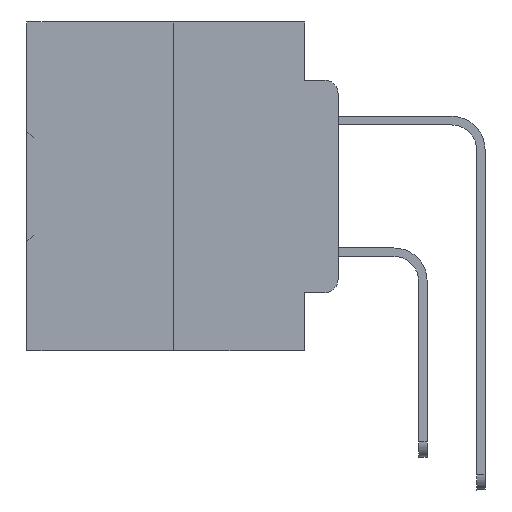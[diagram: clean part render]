
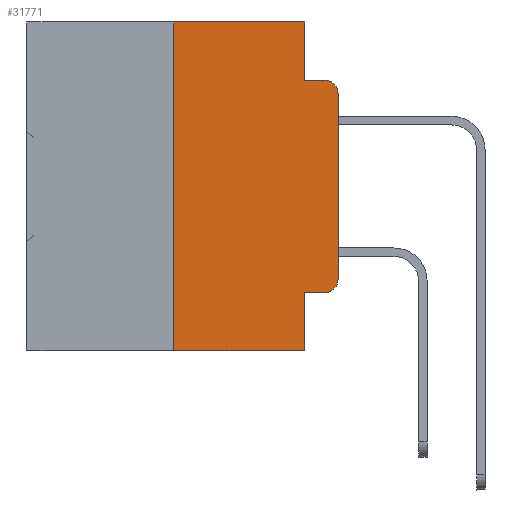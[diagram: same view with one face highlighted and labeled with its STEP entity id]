
A CAD part, left-side view. The second image highlights one B-rep face of the part: STEP entity #31771.
In plain terms, the highlighted planar face has unit normal (-1, 0, 0).
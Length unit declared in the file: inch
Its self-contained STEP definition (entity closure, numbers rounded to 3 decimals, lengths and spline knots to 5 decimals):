
#465 = LINE ( 'NONE', #18030, #31198 ) ;
#1318 = LINE ( 'NONE', #3230, #31983 ) ;
#2475 = DIRECTION ( 'NONE',  ( 0., 0., -1. ) ) ;
#2987 = EDGE_CURVE ( 'NONE', #26139, #19857, #32625, .T. ) ;
#3230 = CARTESIAN_POINT ( 'NONE',  ( 0., 0.25, 0. ) ) ;
#3264 = FACE_OUTER_BOUND ( 'NONE', #35237, .T. ) ;
#4497 = VERTEX_POINT ( 'NONE', #24549 ) ;
#4866 = ORIENTED_EDGE ( 'NONE', *, *, #21084, .F. ) ;
#6070 = DIRECTION ( 'NONE',  ( 0., 0., 1. ) ) ;
#6097 = CARTESIAN_POINT ( 'NONE',  ( 0., 0.051, -0.4115 ) ) ;
#6256 = DIRECTION ( 'NONE',  ( 0., -1., 0. ) ) ;
#6390 = CARTESIAN_POINT ( 'NONE',  ( 0., 0.473, -0.5 ) ) ;
#7211 = ORIENTED_EDGE ( 'NONE', *, *, #20123, .F. ) ;
#7515 = AXIS2_PLACEMENT_3D ( 'NONE', #36043, #9450, #29818 ) ;
#7609 = VECTOR ( 'NONE', #23160, 39.37008 ) ;
#8146 = ORIENTED_EDGE ( 'NONE', *, *, #8311, .F. ) ;
#8180 = LINE ( 'NONE', #6390, #29022 ) ;
#8311 = EDGE_CURVE ( 'NONE', #30500, #19254, #32648, .T. ) ;
#9120 = DIRECTION ( 'NONE',  ( 0., -1., 0. ) ) ;
#9134 = VECTOR ( 'NONE', #10815, 39.37008 ) ;
#9450 = DIRECTION ( 'NONE',  ( -1., 0., 0. ) ) ;
#10042 = ORIENTED_EDGE ( 'NONE', *, *, #34642, .F. ) ;
#10246 = CARTESIAN_POINT ( 'NONE',  ( 0., 0.051, -0.4115 ) ) ;
#10800 = VERTEX_POINT ( 'NONE', #15929 ) ;
#10815 = DIRECTION ( 'NONE',  ( 0., 0., -1. ) ) ;
#12585 = DIRECTION ( 'NONE',  ( 0., -1., 0. ) ) ;
#12762 = CIRCLE ( 'NONE', #13317, 0.02 ) ;
#12876 = ORIENTED_EDGE ( 'NONE', *, *, #13120, .T. ) ;
#13120 = EDGE_CURVE ( 'NONE', #19625, #26139, #36377, .T. ) ;
#13194 = DIRECTION ( 'NONE',  ( -1., 0., 0. ) ) ;
#13317 = AXIS2_PLACEMENT_3D ( 'NONE', #30758, #13194, #33690 ) ;
#13896 = VERTEX_POINT ( 'NONE', #32907 ) ;
#14576 = CARTESIAN_POINT ( 'NONE',  ( 0., 0.02, -0.4115 ) ) ;
#14990 = VECTOR ( 'NONE', #12585, 39.37008 ) ;
#15929 = CARTESIAN_POINT ( 'NONE',  ( 0., 0.051, -0.5 ) ) ;
#18030 = CARTESIAN_POINT ( 'NONE',  ( 0., 0., 0. ) ) ;
#18532 = CARTESIAN_POINT ( 'NONE',  ( 0., 0.02, -0.0885 ) ) ;
#19254 = VERTEX_POINT ( 'NONE', #26486 ) ;
#19493 = VECTOR ( 'NONE', #24830, 39.37008 ) ;
#19625 = VERTEX_POINT ( 'NONE', #10246 ) ;
#19795 = VERTEX_POINT ( 'NONE', #28828 ) ;
#19857 = VERTEX_POINT ( 'NONE', #32105 ) ;
#20123 = EDGE_CURVE ( 'NONE', #19254, #25121, #38294, .T. ) ;
#20477 = DIRECTION ( 'NONE',  ( 1., 0., 0. ) ) ;
#20642 = EDGE_CURVE ( 'NONE', #19857, #13896, #465, .T. ) ;
#21084 = EDGE_CURVE ( 'NONE', #19625, #10800, #31165, .T. ) ;
#23070 = EDGE_CURVE ( 'NONE', #19795, #4497, #1318, .T. ) ;
#23160 = DIRECTION ( 'NONE',  ( 0., 0., -1. ) ) ;
#24549 = CARTESIAN_POINT ( 'NONE',  ( 0., 0.25, 0. ) ) ;
#24830 = DIRECTION ( 'NONE',  ( 0., -1., 0. ) ) ;
#25121 = VERTEX_POINT ( 'NONE', #18532 ) ;
#25343 = AXIS2_PLACEMENT_3D ( 'NONE', #37882, #20477, #2475 ) ;
#25831 = CARTESIAN_POINT ( 'NONE',  ( 0., 0.051, 0. ) ) ;
#25849 = ORIENTED_EDGE ( 'NONE', *, *, #23070, .F. ) ;
#26139 = VERTEX_POINT ( 'NONE', #14576 ) ;
#26312 = EDGE_CURVE ( 'NONE', #19795, #10800, #8180, .T. ) ;
#26486 = CARTESIAN_POINT ( 'NONE',  ( 0., 0.051, -0.0885 ) ) ;
#27195 = ORIENTED_EDGE ( 'NONE', *, *, #20642, .T. ) ;
#27282 = LINE ( 'NONE', #30603, #19493 ) ;
#27302 = CARTESIAN_POINT ( 'NONE',  ( 0., 0.051, -0.0885 ) ) ;
#28070 = ORIENTED_EDGE ( 'NONE', *, *, #37670, .T. ) ;
#28828 = CARTESIAN_POINT ( 'NONE',  ( 0., 0.25, -0.5 ) ) ;
#29022 = VECTOR ( 'NONE', #6256, 39.37008 ) ;
#29818 = DIRECTION ( 'NONE',  ( 0., 0., -1. ) ) ;
#30500 = VERTEX_POINT ( 'NONE', #25831 ) ;
#30603 = CARTESIAN_POINT ( 'NONE',  ( 0., 0.473, 0. ) ) ;
#30758 = CARTESIAN_POINT ( 'NONE',  ( 0., 0.02, -0.1085 ) ) ;
#31165 = LINE ( 'NONE', #37603, #7609 ) ;
#31198 = VECTOR ( 'NONE', #6070, 39.37008 ) ;
#31391 = CARTESIAN_POINT ( 'NONE',  ( 0., 0.051, 0. ) ) ;
#31771 = ADVANCED_FACE ( 'NONE', ( #3264 ), #32039, .F. ) ;
#31983 = VECTOR ( 'NONE', #32881, 39.37008 ) ;
#32039 = PLANE ( 'NONE',  #25343 ) ;
#32105 = CARTESIAN_POINT ( 'NONE',  ( 0., 0., -0.3915 ) ) ;
#32625 = CIRCLE ( 'NONE', #7515, 0.02 ) ;
#32648 = LINE ( 'NONE', #31391, #9134 ) ;
#32881 = DIRECTION ( 'NONE',  ( 0., 0., 1. ) ) ;
#32907 = CARTESIAN_POINT ( 'NONE',  ( 0., 0., -0.1085 ) ) ;
#33505 = ORIENTED_EDGE ( 'NONE', *, *, #26312, .T. ) ;
#33690 = DIRECTION ( 'NONE',  ( 0., 0., -1. ) ) ;
#34642 = EDGE_CURVE ( 'NONE', #4497, #30500, #27282, .T. ) ;
#35237 = EDGE_LOOP ( 'NONE', ( #27195, #28070, #7211, #8146, #10042, #25849, #33505, #4866, #12876, #36250 ) ) ;
#35486 = VECTOR ( 'NONE', #9120, 39.37008 ) ;
#36043 = CARTESIAN_POINT ( 'NONE',  ( 0., 0.02, -0.3915 ) ) ;
#36250 = ORIENTED_EDGE ( 'NONE', *, *, #2987, .T. ) ;
#36377 = LINE ( 'NONE', #6097, #35486 ) ;
#37603 = CARTESIAN_POINT ( 'NONE',  ( 0., 0.051, 0. ) ) ;
#37670 = EDGE_CURVE ( 'NONE', #13896, #25121, #12762, .T. ) ;
#37882 = CARTESIAN_POINT ( 'NONE',  ( 0., 0.473, 0. ) ) ;
#38294 = LINE ( 'NONE', #27302, #14990 ) ;
